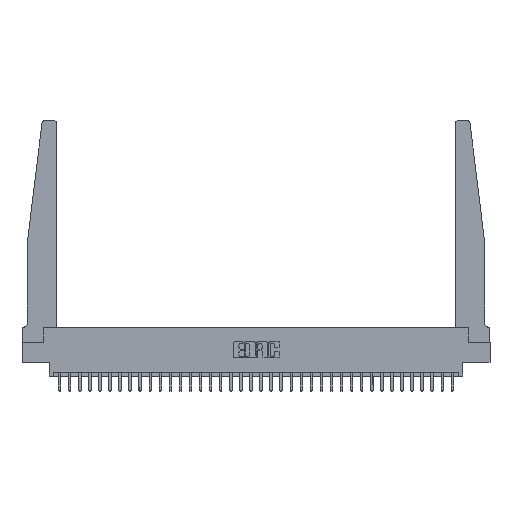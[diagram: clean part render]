
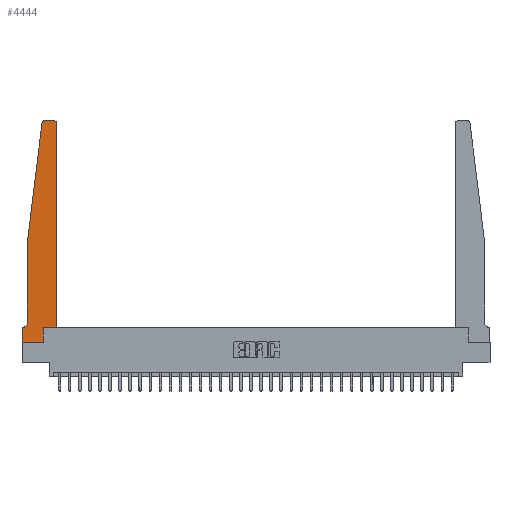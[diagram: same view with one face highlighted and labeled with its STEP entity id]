
A CAD part, top view. The second image highlights one B-rep face of the part: STEP entity #4444.
In plain terms, the highlighted planar face has unit normal (0, 0, 1).
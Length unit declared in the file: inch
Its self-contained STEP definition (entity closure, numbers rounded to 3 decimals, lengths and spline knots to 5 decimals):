
#113 = EDGE_CURVE ( 'NONE', #2832, #20646, #24144, .T. ) ;
#118 = DIRECTION ( 'NONE',  ( 1., 0., 0. ) ) ;
#955 = VERTEX_POINT ( 'NONE', #21744 ) ;
#1045 = DIRECTION ( 'NONE',  ( 0., 1., 0. ) ) ;
#1196 = CARTESIAN_POINT ( 'NONE',  ( 0., 0., 0.37 ) ) ;
#1403 = CARTESIAN_POINT ( 'NONE',  ( 0.2605, 0., 0.37 ) ) ;
#1725 = VECTOR ( 'NONE', #31438, 39.37008 ) ;
#2121 = VERTEX_POINT ( 'NONE', #5176 ) ;
#2507 = DIRECTION ( 'NONE',  ( 1., 0., 0. ) ) ;
#2832 = VERTEX_POINT ( 'NONE', #2858 ) ;
#2858 = CARTESIAN_POINT ( 'NONE',  ( 0.015, 0.1875, 0.37 ) ) ;
#3913 = ORIENTED_EDGE ( 'NONE', *, *, #22292, .T. ) ;
#3919 = VECTOR ( 'NONE', #29137, 39.37008 ) ;
#4349 = ORIENTED_EDGE ( 'NONE', *, *, #24336, .T. ) ;
#4444 = ADVANCED_FACE ( 'NONE', ( #23879 ), #20948, .T. ) ;
#4506 = CARTESIAN_POINT ( 'NONE',  ( 0.065, 1.25, 0.37 ) ) ;
#4893 = DIRECTION ( 'NONE',  ( 0., 0., 1. ) ) ;
#5021 = CARTESIAN_POINT ( 'NONE',  ( 0.065, 0.2375, 0.37 ) ) ;
#5176 = CARTESIAN_POINT ( 'NONE',  ( 0.27653, 2.75, 0.37 ) ) ;
#6162 = CARTESIAN_POINT ( 'NONE',  ( 0.2605, 0.18, 0.37 ) ) ;
#6365 = ORIENTED_EDGE ( 'NONE', *, *, #113, .T. ) ;
#6960 = EDGE_CURVE ( 'NONE', #22708, #19125, #9491, .T. ) ;
#7698 = ORIENTED_EDGE ( 'NONE', *, *, #10157, .T. ) ;
#8549 = EDGE_CURVE ( 'NONE', #2121, #955, #21378, .T. ) ;
#8759 = DIRECTION ( 'NONE',  ( 0., -1., 0. ) ) ;
#9177 = LINE ( 'NONE', #28883, #17481 ) ;
#9491 = CIRCLE ( 'NONE', #27546, 0.03 ) ;
#10013 = AXIS2_PLACEMENT_3D ( 'NONE', #19591, #4893, #2507 ) ;
#10074 = CARTESIAN_POINT ( 'NONE',  ( 0., 0., 0.37 ) ) ;
#10157 = EDGE_CURVE ( 'NONE', #11607, #22708, #11168, .T. ) ;
#10231 = VERTEX_POINT ( 'NONE', #16350 ) ;
#10603 = DIRECTION ( 'NONE',  ( -1., 0., 0. ) ) ;
#10878 = ORIENTED_EDGE ( 'NONE', *, *, #26695, .T. ) ;
#10963 = CARTESIAN_POINT ( 'NONE',  ( 0.395, 2.75, 0.37 ) ) ;
#11092 = DIRECTION ( 'NONE',  ( 1., 0., 0. ) ) ;
#11168 = LINE ( 'NONE', #23123, #14751 ) ;
#11438 = ORIENTED_EDGE ( 'NONE', *, *, #28276, .T. ) ;
#11607 = VERTEX_POINT ( 'NONE', #25268 ) ;
#13487 = ORIENTED_EDGE ( 'NONE', *, *, #27379, .T. ) ;
#13798 = VECTOR ( 'NONE', #8759, 39.37008 ) ;
#14521 = LINE ( 'NONE', #4506, #1725 ) ;
#14598 = EDGE_CURVE ( 'NONE', #19125, #2121, #29765, .T. ) ;
#14751 = VECTOR ( 'NONE', #1045, 39.37008 ) ;
#14923 = DIRECTION ( 'NONE',  ( 1., 0., 0. ) ) ;
#14954 = ORIENTED_EDGE ( 'NONE', *, *, #17441, .T. ) ;
#15070 = CARTESIAN_POINT ( 'NONE',  ( 0., 0., 0.37 ) ) ;
#15420 = VERTEX_POINT ( 'NONE', #10074 ) ;
#15649 = EDGE_LOOP ( 'NONE', ( #19345, #17133, #11438, #30593, #3913, #6365, #14954, #13487, #10878, #4349, #7698, #31388 ) ) ;
#16350 = CARTESIAN_POINT ( 'NONE',  ( 0.065, 1.25, 0.37 ) ) ;
#17043 = CARTESIAN_POINT ( 'NONE',  ( 0.25, 2.75, 0.37 ) ) ;
#17133 = ORIENTED_EDGE ( 'NONE', *, *, #8549, .T. ) ;
#17441 = EDGE_CURVE ( 'NONE', #20646, #15420, #20846, .T. ) ;
#17481 = VECTOR ( 'NONE', #29029, 39.37008 ) ;
#17502 = DIRECTION ( 'NONE',  ( -1., 0., 0. ) ) ;
#17752 = CARTESIAN_POINT ( 'NONE',  ( 0., 0.1875, 0.37 ) ) ;
#17892 = CARTESIAN_POINT ( 'NONE',  ( 0.015, 0.2375, 0.37 ) ) ;
#18089 = CARTESIAN_POINT ( 'NONE',  ( 0.2605, 0.18, 0.37 ) ) ;
#18133 = VERTEX_POINT ( 'NONE', #1403 ) ;
#18970 = VECTOR ( 'NONE', #25112, 39.37008 ) ;
#19125 = VERTEX_POINT ( 'NONE', #10963 ) ;
#19279 = CARTESIAN_POINT ( 'NONE',  ( 0.065, 0.1875, 0.37 ) ) ;
#19345 = ORIENTED_EDGE ( 'NONE', *, *, #14598, .T. ) ;
#19591 = CARTESIAN_POINT ( 'NONE',  ( 0.27653, 2.72, 0.37 ) ) ;
#20459 = VERTEX_POINT ( 'NONE', #5021 ) ;
#20633 = DIRECTION ( 'NONE',  ( 0., 0., -1. ) ) ;
#20646 = VERTEX_POINT ( 'NONE', #17752 ) ;
#20846 = LINE ( 'NONE', #1196, #13798 ) ;
#20948 = PLANE ( 'NONE',  #29632 ) ;
#21378 = CIRCLE ( 'NONE', #10013, 0.03 ) ;
#21744 = CARTESIAN_POINT ( 'NONE',  ( 0.24675, 2.72367, 0.37 ) ) ;
#22292 = EDGE_CURVE ( 'NONE', #20459, #2832, #31805, .T. ) ;
#22708 = VERTEX_POINT ( 'NONE', #22848 ) ;
#22848 = CARTESIAN_POINT ( 'NONE',  ( 0.425, 2.72, 0.37 ) ) ;
#23047 = AXIS2_PLACEMENT_3D ( 'NONE', #17892, #20633, #10603 ) ;
#23123 = CARTESIAN_POINT ( 'NONE',  ( 0.425, 0.18, 0.37 ) ) ;
#23221 = DIRECTION ( 'NONE',  ( 0., 0., 1. ) ) ;
#23879 = FACE_OUTER_BOUND ( 'NONE', #15649, .T. ) ;
#24144 = LINE ( 'NONE', #19279, #3919 ) ;
#24233 = CARTESIAN_POINT ( 'NONE',  ( 0.065, 1.25, 0.37 ) ) ;
#24336 = EDGE_CURVE ( 'NONE', #29403, #11607, #9177, .T. ) ;
#24794 = DIRECTION ( 'NONE',  ( 0., 0., 1. ) ) ;
#25112 = DIRECTION ( 'NONE',  ( -0.122, -0.992, 0. ) ) ;
#25268 = CARTESIAN_POINT ( 'NONE',  ( 0.425, 0.18, 0.37 ) ) ;
#25403 = CARTESIAN_POINT ( 'NONE',  ( 0.395, 2.72, 0.37 ) ) ;
#25567 = VECTOR ( 'NONE', #17502, 39.37008 ) ;
#25852 = DIRECTION ( 'NONE',  ( 0., 1., 0. ) ) ;
#25864 = VECTOR ( 'NONE', #14923, 39.37008 ) ;
#26695 = EDGE_CURVE ( 'NONE', #18133, #29403, #28294, .T. ) ;
#27183 = LINE ( 'NONE', #15070, #25864 ) ;
#27379 = EDGE_CURVE ( 'NONE', #15420, #18133, #27183, .T. ) ;
#27546 = AXIS2_PLACEMENT_3D ( 'NONE', #25403, #24794, #118 ) ;
#27886 = VECTOR ( 'NONE', #25852, 39.37008 ) ;
#28276 = EDGE_CURVE ( 'NONE', #955, #10231, #29946, .T. ) ;
#28294 = LINE ( 'NONE', #6162, #27886 ) ;
#28883 = CARTESIAN_POINT ( 'NONE',  ( 0.425, 0.18, 0.37 ) ) ;
#29029 = DIRECTION ( 'NONE',  ( 1., 0., 0. ) ) ;
#29137 = DIRECTION ( 'NONE',  ( -1., 0., 0. ) ) ;
#29403 = VERTEX_POINT ( 'NONE', #18089 ) ;
#29632 = AXIS2_PLACEMENT_3D ( 'NONE', #31113, #23221, #11092 ) ;
#29765 = LINE ( 'NONE', #17043, #25567 ) ;
#29946 = LINE ( 'NONE', #24233, #18970 ) ;
#30593 = ORIENTED_EDGE ( 'NONE', *, *, #31427, .T. ) ;
#31113 = CARTESIAN_POINT ( 'NONE',  ( 0., 0.1875, 0.37 ) ) ;
#31388 = ORIENTED_EDGE ( 'NONE', *, *, #6960, .T. ) ;
#31427 = EDGE_CURVE ( 'NONE', #10231, #20459, #14521, .T. ) ;
#31438 = DIRECTION ( 'NONE',  ( 0., -1., 0. ) ) ;
#31805 = CIRCLE ( 'NONE', #23047, 0.05 ) ;
